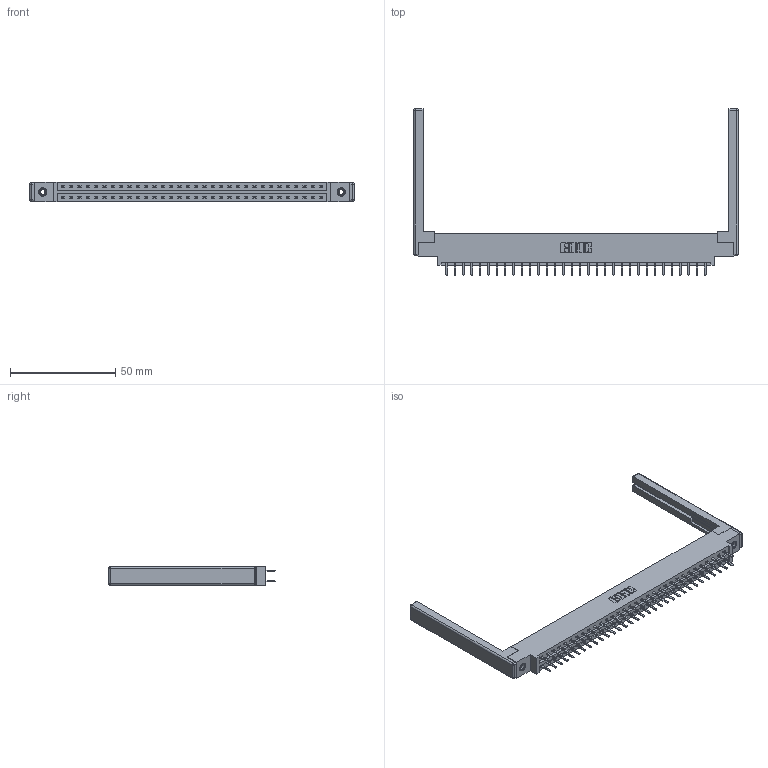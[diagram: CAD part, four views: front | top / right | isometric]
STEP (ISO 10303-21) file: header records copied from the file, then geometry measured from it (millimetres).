
FILE_DESCRIPTION (( 'STEP AP203' ), '1' );
FILE_NAME ('337-064-520-868.STEP', '2019-10-11T23:28:15', ( '' ), ( '' ), 'SwSTEP 2.0', 'SolidWorks 2016', '' );
FILE_SCHEMA (( 'CONFIG_CONTROL_DESIGN' ));
Length unit declared in the file: inch
Products named in the file (5): 345-250-001_345-250-001-102; 337 Part_0.170 Offset - 0.156 Dia-TI; 345-292-001_345-293-120; 307-220-068; 337-064-520-868
Assembly tree (69 placements, depth 2):
  337-064-520-868
    337 Part_0.170 Offset - 0.156 Dia-TI
    345-292-001_345-293-120  x64
    345-250-001_345-250-001-102  x2
    307-220-068  x2
Bounding box: 154.23 x 79.08 x 9.4 mm (x, y, z)
Volume: 20359.9 mm3; surface area: 22024.7 mm2
Topology: 69 solids, 69 shells, 3984 faces, 11529 edges, 7494 vertices
Faces by surface type: plane 2722, cylinder 1238, cone 12, sphere 8, torus 4
Entity records: 29110 total; most frequent: CARTESIAN_POINT 4891, ORIENTED_EDGE 4804, DIRECTION 4236, EDGE_CURVE 2402, LINE 2220, VECTOR 2220, VERTEX_POINT 1590, AXIS2_PLACEMENT_3D 1008
